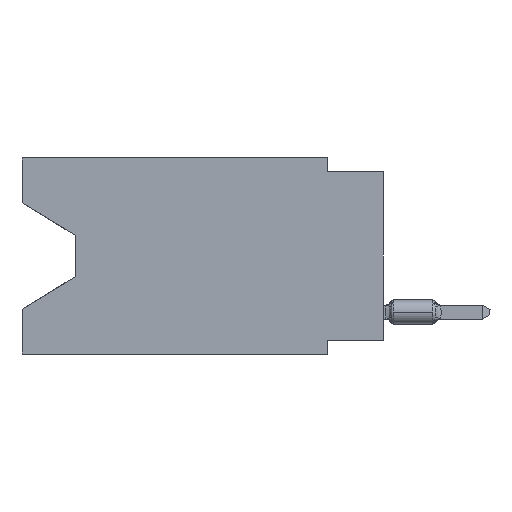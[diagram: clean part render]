
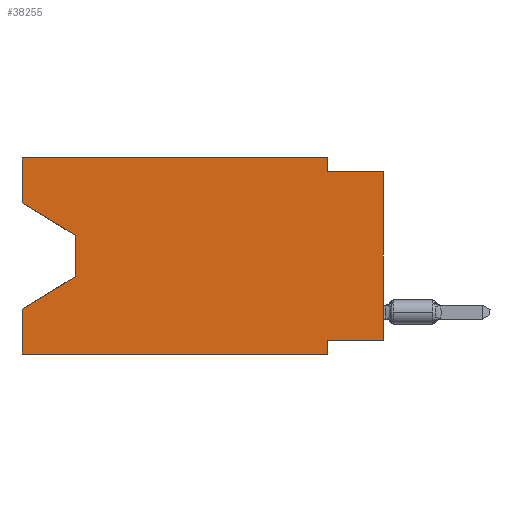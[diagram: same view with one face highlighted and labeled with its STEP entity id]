
A CAD part, left-side view. The second image highlights one B-rep face of the part: STEP entity #38255.
In plain terms, the highlighted planar face has unit normal (-1, 0, 0).
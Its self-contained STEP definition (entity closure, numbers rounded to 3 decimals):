
#640 = ORIENTED_EDGE ( 'NONE', *, *, #23621, .F. ) ;
#933 = EDGE_CURVE ( 'NONE', #12241, #37597, #24105, .T. ) ;
#1367 = EDGE_CURVE ( 'NONE', #19468, #35296, #36189, .T. ) ;
#1833 = EDGE_CURVE ( 'NONE', #16210, #11212, #27959, .T. ) ;
#2085 = VECTOR ( 'NONE', #35265, 1000. ) ;
#3525 = CARTESIAN_POINT ( 'NONE',  ( 0., 0., -0.635 ) ) ;
#3657 = DIRECTION ( 'NONE',  ( 0., -1., 0. ) ) ;
#4411 = VECTOR ( 'NONE', #16327, 1000. ) ;
#4814 = DIRECTION ( 'NONE',  ( 0., 0., -1. ) ) ;
#5169 = LINE ( 'NONE', #13615, #5305 ) ;
#5305 = VECTOR ( 'NONE', #18081, 1000. ) ;
#5497 = AXIS2_PLACEMENT_3D ( 'NONE', #38023, #49351, #37757 ) ;
#5589 = EDGE_CURVE ( 'NONE', #14032, #12241, #5169, .T. ) ;
#5835 = DIRECTION ( 'NONE',  ( 0., 0., 1. ) ) ;
#6236 = CARTESIAN_POINT ( 'NONE',  ( 0., 13.97, -3.505 ) ) ;
#6431 = LINE ( 'NONE', #26265, #27905 ) ;
#7516 = EDGE_CURVE ( 'NONE', #18215, #15568, #10786, .T. ) ;
#7678 = EDGE_CURVE ( 'NONE', #15883, #16210, #37439, .T. ) ;
#7893 = VERTEX_POINT ( 'NONE', #14436 ) ;
#8957 = ORIENTED_EDGE ( 'NONE', *, *, #51505, .T. ) ;
#9513 = EDGE_CURVE ( 'NONE', #11212, #7893, #30536, .T. ) ;
#10644 = CARTESIAN_POINT ( 'NONE',  ( 0., 2.54, 0. ) ) ;
#10786 = LINE ( 'NONE', #40098, #15540 ) ;
#11212 = VERTEX_POINT ( 'NONE', #18386 ) ;
#11936 = ORIENTED_EDGE ( 'NONE', *, *, #35581, .F. ) ;
#12241 = VERTEX_POINT ( 'NONE', #12960 ) ;
#12960 = CARTESIAN_POINT ( 'NONE',  ( 0., 2.54, -0.635 ) ) ;
#13615 = CARTESIAN_POINT ( 'NONE',  ( 0., 2.54, 0. ) ) ;
#14032 = VERTEX_POINT ( 'NONE', #10644 ) ;
#14090 = VECTOR ( 'NONE', #4814, 1000. ) ;
#14436 = CARTESIAN_POINT ( 'NONE',  ( 0., 16.383, -6.852 ) ) ;
#14476 = VECTOR ( 'NONE', #5835, 1000. ) ;
#15540 = VECTOR ( 'NONE', #3657, 1000. ) ;
#15568 = VERTEX_POINT ( 'NONE', #42207 ) ;
#15604 = DIRECTION ( 'NONE',  ( 0., 1., 0. ) ) ;
#15798 = LINE ( 'NONE', #16594, #4411 ) ;
#15883 = VERTEX_POINT ( 'NONE', #36630 ) ;
#16210 = VERTEX_POINT ( 'NONE', #6236 ) ;
#16327 = DIRECTION ( 'NONE',  ( 0., 0., 1. ) ) ;
#16501 = CARTESIAN_POINT ( 'NONE',  ( 0., 16.383, -8.89 ) ) ;
#16594 = CARTESIAN_POINT ( 'NONE',  ( 0., 0., 0. ) ) ;
#17048 = CARTESIAN_POINT ( 'NONE',  ( 0., 16.383, 0. ) ) ;
#18081 = DIRECTION ( 'NONE',  ( 0., 0., -1. ) ) ;
#18215 = VERTEX_POINT ( 'NONE', #16501 ) ;
#18386 = CARTESIAN_POINT ( 'NONE',  ( 0., 13.97, -5.385 ) ) ;
#19468 = VERTEX_POINT ( 'NONE', #40418 ) ;
#19754 = CARTESIAN_POINT ( 'NONE',  ( 0., 13.97, -3.505 ) ) ;
#23123 = CARTESIAN_POINT ( 'NONE',  ( 0., 0., -0.635 ) ) ;
#23621 = EDGE_CURVE ( 'NONE', #35296, #15568, #28325, .T. ) ;
#24105 = LINE ( 'NONE', #3525, #40313 ) ;
#24740 = ORIENTED_EDGE ( 'NONE', *, *, #9513, .T. ) ;
#26265 = CARTESIAN_POINT ( 'NONE',  ( 0., 16.383, 0. ) ) ;
#26700 = DIRECTION ( 'NONE',  ( 0., 0., 1. ) ) ;
#27905 = VECTOR ( 'NONE', #38651, 1000. ) ;
#27959 = LINE ( 'NONE', #19754, #52117 ) ;
#28325 = LINE ( 'NONE', #40977, #14090 ) ;
#28502 = ORIENTED_EDGE ( 'NONE', *, *, #7516, .T. ) ;
#29257 = DIRECTION ( 'NONE',  ( 0., -0.855, -0.519 ) ) ;
#29313 = PLANE ( 'NONE',  #5497 ) ;
#30536 = LINE ( 'NONE', #34486, #2085 ) ;
#30765 = ORIENTED_EDGE ( 'NONE', *, *, #1367, .F. ) ;
#30905 = ORIENTED_EDGE ( 'NONE', *, *, #5589, .F. ) ;
#31712 = CARTESIAN_POINT ( 'NONE',  ( 0., 0., -8.255 ) ) ;
#33345 = EDGE_CURVE ( 'NONE', #15883, #39056, #33816, .T. ) ;
#33816 = LINE ( 'NONE', #50156, #14476 ) ;
#34242 = CARTESIAN_POINT ( 'NONE',  ( 0., 16.383, -2.038 ) ) ;
#34486 = CARTESIAN_POINT ( 'NONE',  ( 0., 13.97, -5.385 ) ) ;
#35265 = DIRECTION ( 'NONE',  ( 0., 0.855, -0.519 ) ) ;
#35296 = VERTEX_POINT ( 'NONE', #38896 ) ;
#35350 = DIRECTION ( 'NONE',  ( 0., 0., -1. ) ) ;
#35581 = EDGE_CURVE ( 'NONE', #18215, #7893, #43287, .T. ) ;
#36189 = LINE ( 'NONE', #31712, #36994 ) ;
#36630 = CARTESIAN_POINT ( 'NONE',  ( 0., 16.383, -2.038 ) ) ;
#36994 = VECTOR ( 'NONE', #15604, 1000. ) ;
#37207 = ORIENTED_EDGE ( 'NONE', *, *, #933, .F. ) ;
#37439 = LINE ( 'NONE', #34242, #47488 ) ;
#37484 = ORIENTED_EDGE ( 'NONE', *, *, #1833, .T. ) ;
#37597 = VERTEX_POINT ( 'NONE', #23123 ) ;
#37757 = DIRECTION ( 'NONE',  ( 0., 0., -1. ) ) ;
#37784 = ORIENTED_EDGE ( 'NONE', *, *, #46738, .F. ) ;
#38023 = CARTESIAN_POINT ( 'NONE',  ( 0., 16.383, 0. ) ) ;
#38255 = ADVANCED_FACE ( 'NONE', ( #38523 ), #29313, .F. ) ;
#38523 = FACE_OUTER_BOUND ( 'NONE', #49197, .T. ) ;
#38651 = DIRECTION ( 'NONE',  ( 0., -1., 0. ) ) ;
#38896 = CARTESIAN_POINT ( 'NONE',  ( 0., 2.54, -8.255 ) ) ;
#39056 = VERTEX_POINT ( 'NONE', #17048 ) ;
#40098 = CARTESIAN_POINT ( 'NONE',  ( 0., 16.383, -8.89 ) ) ;
#40226 = DIRECTION ( 'NONE',  ( 0., -1., 0. ) ) ;
#40313 = VECTOR ( 'NONE', #40226, 1000. ) ;
#40418 = CARTESIAN_POINT ( 'NONE',  ( 0., 0., -8.255 ) ) ;
#40773 = ORIENTED_EDGE ( 'NONE', *, *, #33345, .F. ) ;
#40977 = CARTESIAN_POINT ( 'NONE',  ( 0., 2.54, -8.89 ) ) ;
#42207 = CARTESIAN_POINT ( 'NONE',  ( 0., 2.54, -8.89 ) ) ;
#43287 = LINE ( 'NONE', #50421, #45848 ) ;
#45616 = ORIENTED_EDGE ( 'NONE', *, *, #7678, .T. ) ;
#45848 = VECTOR ( 'NONE', #26700, 1000. ) ;
#46738 = EDGE_CURVE ( 'NONE', #39056, #14032, #6431, .T. ) ;
#47488 = VECTOR ( 'NONE', #29257, 1000. ) ;
#49197 = EDGE_LOOP ( 'NONE', ( #45616, #37484, #24740, #11936, #28502, #640, #30765, #8957, #37207, #30905, #37784, #40773 ) ) ;
#49351 = DIRECTION ( 'NONE',  ( 1., 0., 0. ) ) ;
#50156 = CARTESIAN_POINT ( 'NONE',  ( 0., 16.383, 0. ) ) ;
#50421 = CARTESIAN_POINT ( 'NONE',  ( 0., 16.383, 0. ) ) ;
#51505 = EDGE_CURVE ( 'NONE', #19468, #37597, #15798, .T. ) ;
#52117 = VECTOR ( 'NONE', #35350, 1000. ) ;
